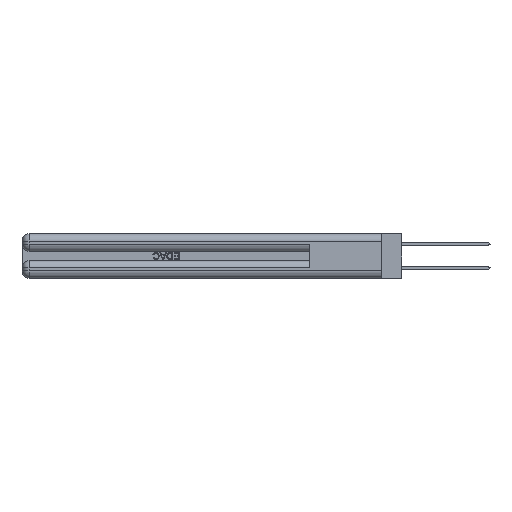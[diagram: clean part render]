
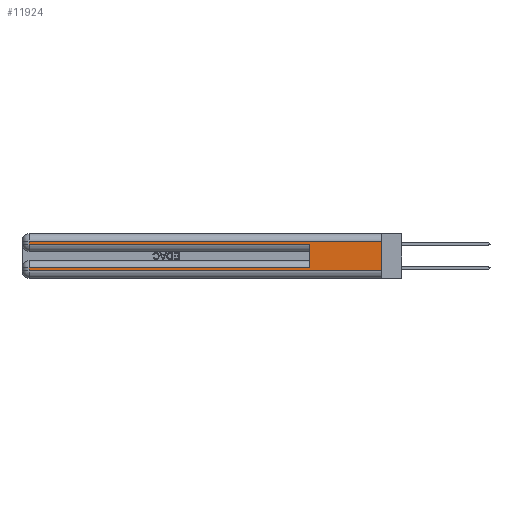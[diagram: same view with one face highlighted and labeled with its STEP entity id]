
A CAD part, left-side view. The second image highlights one B-rep face of the part: STEP entity #11924.
In plain terms, the highlighted planar face has unit normal (-1, 0, 0).
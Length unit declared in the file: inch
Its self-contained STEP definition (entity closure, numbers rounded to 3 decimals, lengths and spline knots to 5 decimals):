
#262 = VECTOR ( 'NONE', #1316, 39.37008 ) ;
#477 = VERTEX_POINT ( 'NONE', #42956 ) ;
#1316 = DIRECTION ( 'NONE',  ( 0., 0., -1. ) ) ;
#1649 = ORIENTED_EDGE ( 'NONE', *, *, #8162, .T. ) ;
#2096 = ORIENTED_EDGE ( 'NONE', *, *, #46078, .F. ) ;
#2240 = FACE_OUTER_BOUND ( 'NONE', #42120, .T. ) ;
#2508 = CARTESIAN_POINT ( 'NONE',  ( 0., 0., 0.31 ) ) ;
#2982 = CARTESIAN_POINT ( 'NONE',  ( 0., 0., 0.31 ) ) ;
#3380 = LINE ( 'NONE', #11656, #41511 ) ;
#3409 = VECTOR ( 'NONE', #36380, 39.37008 ) ;
#3438 = AXIS2_PLACEMENT_3D ( 'NONE', #3539, #14648, #40538 ) ;
#3539 = CARTESIAN_POINT ( 'NONE',  ( 0., 0., 0.37 ) ) ;
#4530 = ORIENTED_EDGE ( 'NONE', *, *, #8858, .T. ) ;
#5004 = EDGE_CURVE ( 'NONE', #37023, #21503, #45654, .T. ) ;
#6577 = LINE ( 'NONE', #33327, #15230 ) ;
#7339 = ORIENTED_EDGE ( 'NONE', *, *, #40079, .T. ) ;
#8162 = EDGE_CURVE ( 'NONE', #37023, #32934, #42421, .T. ) ;
#8858 = EDGE_CURVE ( 'NONE', #32934, #45936, #6577, .T. ) ;
#8893 = CARTESIAN_POINT ( 'NONE',  ( 0., 0., 0.06 ) ) ;
#11656 = CARTESIAN_POINT ( 'NONE',  ( 0., 0., 0.085 ) ) ;
#11924 = ADVANCED_FACE ( 'NONE', ( #2240 ), #25666, .F. ) ;
#12227 = CARTESIAN_POINT ( 'NONE',  ( 0., 2.94, 0.37 ) ) ;
#13985 = DIRECTION ( 'NONE',  ( 0., 0., -1. ) ) ;
#14252 = DIRECTION ( 'NONE',  ( 0., 1., 0. ) ) ;
#14648 = DIRECTION ( 'NONE',  ( 1., 0., 0. ) ) ;
#14813 = DIRECTION ( 'NONE',  ( 0., -1., 0. ) ) ;
#15201 = EDGE_CURVE ( 'NONE', #45936, #31038, #23404, .T. ) ;
#15230 = VECTOR ( 'NONE', #40778, 39.37008 ) ;
#18519 = CARTESIAN_POINT ( 'NONE',  ( 0., 0., 0.285 ) ) ;
#21270 = CARTESIAN_POINT ( 'NONE',  ( 0., 0., 0.37 ) ) ;
#21483 = ORIENTED_EDGE ( 'NONE', *, *, #43249, .T. ) ;
#21503 = VERTEX_POINT ( 'NONE', #8893 ) ;
#23318 = CARTESIAN_POINT ( 'NONE',  ( 0., 2.94, 0.085 ) ) ;
#23404 = LINE ( 'NONE', #18519, #41942 ) ;
#24828 = ORIENTED_EDGE ( 'NONE', *, *, #5004, .F. ) ;
#25666 = PLANE ( 'NONE',  #3438 ) ;
#26010 = VECTOR ( 'NONE', #13985, 39.37008 ) ;
#26055 = VERTEX_POINT ( 'NONE', #26221 ) ;
#26221 = CARTESIAN_POINT ( 'NONE',  ( 0., 2.94, 0.06 ) ) ;
#26563 = DIRECTION ( 'NONE',  ( 0., 1., 0. ) ) ;
#29751 = LINE ( 'NONE', #12227, #262 ) ;
#30268 = CARTESIAN_POINT ( 'NONE',  ( 0., 2.94, 0.31 ) ) ;
#31038 = VERTEX_POINT ( 'NONE', #44211 ) ;
#32005 = CARTESIAN_POINT ( 'NONE',  ( 0., 0.6, 0.145 ) ) ;
#32585 = VECTOR ( 'NONE', #14252, 39.37008 ) ;
#32885 = LINE ( 'NONE', #43680, #3409 ) ;
#32934 = VERTEX_POINT ( 'NONE', #30268 ) ;
#33327 = CARTESIAN_POINT ( 'NONE',  ( 0., 2.94, 0.37 ) ) ;
#34448 = ORIENTED_EDGE ( 'NONE', *, *, #15201, .T. ) ;
#35713 = DIRECTION ( 'NONE',  ( 0., 0., 1. ) ) ;
#36380 = DIRECTION ( 'NONE',  ( 0., -1., 0. ) ) ;
#37023 = VERTEX_POINT ( 'NONE', #2982 ) ;
#37340 = LINE ( 'NONE', #32005, #38505 ) ;
#38504 = VERTEX_POINT ( 'NONE', #23318 ) ;
#38505 = VECTOR ( 'NONE', #35713, 39.37008 ) ;
#39358 = EDGE_CURVE ( 'NONE', #477, #38504, #3380, .T. ) ;
#40079 = EDGE_CURVE ( 'NONE', #38504, #26055, #29751, .T. ) ;
#40435 = ORIENTED_EDGE ( 'NONE', *, *, #39358, .T. ) ;
#40538 = DIRECTION ( 'NONE',  ( 0., 0., -1. ) ) ;
#40778 = DIRECTION ( 'NONE',  ( 0., 0., -1. ) ) ;
#41511 = VECTOR ( 'NONE', #26563, 39.37008 ) ;
#41942 = VECTOR ( 'NONE', #14813, 39.37008 ) ;
#42120 = EDGE_LOOP ( 'NONE', ( #24828, #1649, #4530, #34448, #2096, #40435, #7339, #21483 ) ) ;
#42421 = LINE ( 'NONE', #2508, #32585 ) ;
#42956 = CARTESIAN_POINT ( 'NONE',  ( 0., 0.6, 0.085 ) ) ;
#43249 = EDGE_CURVE ( 'NONE', #26055, #21503, #32885, .T. ) ;
#43680 = CARTESIAN_POINT ( 'NONE',  ( 0., 0., 0.06 ) ) ;
#44211 = CARTESIAN_POINT ( 'NONE',  ( 0., 0.6, 0.285 ) ) ;
#45654 = LINE ( 'NONE', #21270, #26010 ) ;
#45904 = CARTESIAN_POINT ( 'NONE',  ( 0., 2.94, 0.285 ) ) ;
#45936 = VERTEX_POINT ( 'NONE', #45904 ) ;
#46078 = EDGE_CURVE ( 'NONE', #477, #31038, #37340, .T. ) ;
